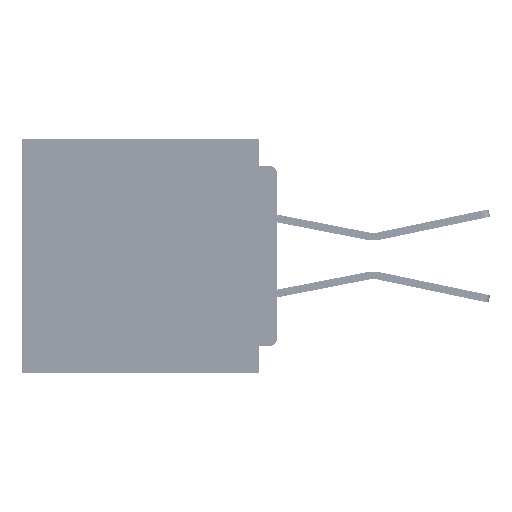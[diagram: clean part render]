
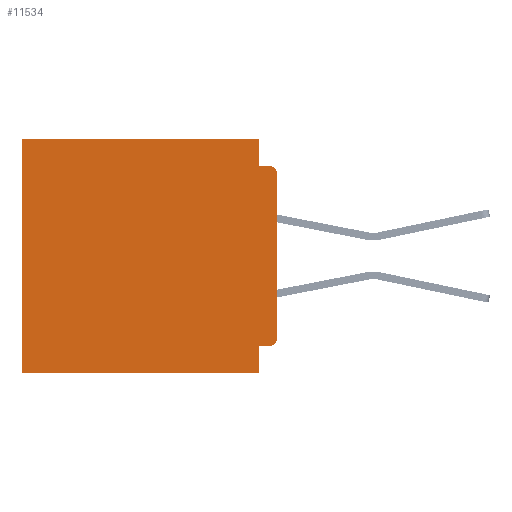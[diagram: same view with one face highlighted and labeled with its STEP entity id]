
A CAD part, left-side view. The second image highlights one B-rep face of the part: STEP entity #11534.
In plain terms, the highlighted planar face has unit normal (-1, 0, 0).
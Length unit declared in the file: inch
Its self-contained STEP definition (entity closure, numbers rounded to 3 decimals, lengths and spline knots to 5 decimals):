
#200 = EDGE_CURVE ( 'NONE', #4685, #11992, #20546, .T. ) ;
#684 = EDGE_LOOP ( 'NONE', ( #48535, #51566, #18633, #61626, #24352, #9855, #30431, #48589, #23209, #20955 ) ) ;
#1313 = VECTOR ( 'NONE', #10297, 39.37008 ) ;
#1827 = DIRECTION ( 'NONE',  ( 0., 0., -1. ) ) ;
#3111 = VECTOR ( 'NONE', #33358, 39.37008 ) ;
#3542 = VECTOR ( 'NONE', #47711, 39.37008 ) ;
#4681 = DIRECTION ( 'NONE',  ( 0., 0., -1. ) ) ;
#4685 = VERTEX_POINT ( 'NONE', #29439 ) ;
#4768 = CIRCLE ( 'NONE', #56144, 0.015 ) ;
#6121 = CARTESIAN_POINT ( 'NONE',  ( 0.3, 0., -0.355 ) ) ;
#6605 = LINE ( 'NONE', #52611, #3542 ) ;
#6770 = CARTESIAN_POINT ( 'NONE',  ( 0.3, 0.031, -0.4 ) ) ;
#7373 = VECTOR ( 'NONE', #21835, 39.37008 ) ;
#7775 = DIRECTION ( 'NONE',  ( -1., 0., 0. ) ) ;
#8286 = PLANE ( 'NONE',  #23350 ) ;
#9855 = ORIENTED_EDGE ( 'NONE', *, *, #56102, .T. ) ;
#10297 = DIRECTION ( 'NONE',  ( 0., 1., 0. ) ) ;
#11070 = DIRECTION ( 'NONE',  ( 0., 1., 0. ) ) ;
#11534 = ADVANCED_FACE ( 'NONE', ( #23353 ), #8286, .F. ) ;
#11992 = VERTEX_POINT ( 'NONE', #26551 ) ;
#13251 = DIRECTION ( 'NONE',  ( 0., 0., -1. ) ) ;
#17113 = VECTOR ( 'NONE', #4681, 39.37008 ) ;
#18633 = ORIENTED_EDGE ( 'NONE', *, *, #31540, .F. ) ;
#18868 = EDGE_CURVE ( 'NONE', #61785, #51885, #62265, .T. ) ;
#19037 = CARTESIAN_POINT ( 'NONE',  ( 0.3, 0.015, -0.355 ) ) ;
#19326 = VERTEX_POINT ( 'NONE', #39690 ) ;
#20546 = LINE ( 'NONE', #61941, #7373 ) ;
#20955 = ORIENTED_EDGE ( 'NONE', *, *, #57345, .T. ) ;
#21835 = DIRECTION ( 'NONE',  ( 0., 1., 0. ) ) ;
#22957 = DIRECTION ( 'NONE',  ( -1., 0., 0. ) ) ;
#23168 = VECTOR ( 'NONE', #1827, 39.37008 ) ;
#23209 = ORIENTED_EDGE ( 'NONE', *, *, #48322, .F. ) ;
#23350 = AXIS2_PLACEMENT_3D ( 'NONE', #32878, #42712, #13251 ) ;
#23353 = FACE_OUTER_BOUND ( 'NONE', #684, .T. ) ;
#24352 = ORIENTED_EDGE ( 'NONE', *, *, #200, .T. ) ;
#25159 = VERTEX_POINT ( 'NONE', #54789 ) ;
#26551 = CARTESIAN_POINT ( 'NONE',  ( 0.3, 0.437, 0. ) ) ;
#27197 = LINE ( 'NONE', #6121, #51786 ) ;
#28138 = VERTEX_POINT ( 'NONE', #58748 ) ;
#29439 = CARTESIAN_POINT ( 'NONE',  ( 0.3, 0.031, 0. ) ) ;
#30431 = ORIENTED_EDGE ( 'NONE', *, *, #61529, .F. ) ;
#31540 = EDGE_CURVE ( 'NONE', #25159, #48718, #52316, .T. ) ;
#32878 = CARTESIAN_POINT ( 'NONE',  ( 0.3, 0., -0.4 ) ) ;
#33358 = DIRECTION ( 'NONE',  ( 0., -1., 0. ) ) ;
#34223 = CARTESIAN_POINT ( 'NONE',  ( 0.3, 0.031, 0. ) ) ;
#37297 = CARTESIAN_POINT ( 'NONE',  ( 0.3, 0.015, -0.06 ) ) ;
#39300 = CARTESIAN_POINT ( 'NONE',  ( 0.3, 0.015, -0.045 ) ) ;
#39690 = CARTESIAN_POINT ( 'NONE',  ( 0.3, 0.437, -0.4 ) ) ;
#40613 = LINE ( 'NONE', #59213, #1313 ) ;
#42242 = DIRECTION ( 'NONE',  ( 0., 0., -1. ) ) ;
#42439 = CARTESIAN_POINT ( 'NONE',  ( 0.3, 0.437, -0.4 ) ) ;
#42663 = VECTOR ( 'NONE', #52264, 39.37008 ) ;
#42712 = DIRECTION ( 'NONE',  ( 1., 0., 0. ) ) ;
#43287 = LINE ( 'NONE', #34223, #17113 ) ;
#45875 = EDGE_CURVE ( 'NONE', #4685, #25159, #43287, .T. ) ;
#46806 = EDGE_CURVE ( 'NONE', #49219, #48718, #4768, .T. ) ;
#47711 = DIRECTION ( 'NONE',  ( 0., 0., -1. ) ) ;
#48322 = EDGE_CURVE ( 'NONE', #60712, #61785, #27197, .T. ) ;
#48535 = ORIENTED_EDGE ( 'NONE', *, *, #55244, .F. ) ;
#48589 = ORIENTED_EDGE ( 'NONE', *, *, #18868, .F. ) ;
#48718 = VERTEX_POINT ( 'NONE', #39300 ) ;
#49219 = VERTEX_POINT ( 'NONE', #57759 ) ;
#50920 = CARTESIAN_POINT ( 'NONE',  ( 0.3, 0.031, -0.4 ) ) ;
#51566 = ORIENTED_EDGE ( 'NONE', *, *, #46806, .T. ) ;
#51721 = CIRCLE ( 'NONE', #53637, 0.015 ) ;
#51786 = VECTOR ( 'NONE', #11070, 39.37008 ) ;
#51885 = VERTEX_POINT ( 'NONE', #50920 ) ;
#52264 = DIRECTION ( 'NONE',  ( 0., 0., -1. ) ) ;
#52316 = LINE ( 'NONE', #57700, #3111 ) ;
#52351 = CARTESIAN_POINT ( 'NONE',  ( 0.3, 0.015, -0.34 ) ) ;
#52611 = CARTESIAN_POINT ( 'NONE',  ( 0.3, 0., -0.4 ) ) ;
#53637 = AXIS2_PLACEMENT_3D ( 'NONE', #52351, #22957, #57220 ) ;
#54789 = CARTESIAN_POINT ( 'NONE',  ( 0.3, 0.031, -0.045 ) ) ;
#55244 = EDGE_CURVE ( 'NONE', #49219, #28138, #6605, .T. ) ;
#55645 = LINE ( 'NONE', #42439, #42663 ) ;
#56102 = EDGE_CURVE ( 'NONE', #11992, #19326, #55645, .T. ) ;
#56144 = AXIS2_PLACEMENT_3D ( 'NONE', #37297, #7775, #42242 ) ;
#57220 = DIRECTION ( 'NONE',  ( 0., 0., -1. ) ) ;
#57345 = EDGE_CURVE ( 'NONE', #60712, #28138, #51721, .T. ) ;
#57700 = CARTESIAN_POINT ( 'NONE',  ( 0.3, 0., -0.045 ) ) ;
#57759 = CARTESIAN_POINT ( 'NONE',  ( 0.3, 0., -0.06 ) ) ;
#58748 = CARTESIAN_POINT ( 'NONE',  ( 0.3, 0., -0.34 ) ) ;
#59213 = CARTESIAN_POINT ( 'NONE',  ( 0.3, 0., -0.4 ) ) ;
#60712 = VERTEX_POINT ( 'NONE', #19037 ) ;
#61384 = CARTESIAN_POINT ( 'NONE',  ( 0.3, 0.031, -0.355 ) ) ;
#61529 = EDGE_CURVE ( 'NONE', #51885, #19326, #40613, .T. ) ;
#61626 = ORIENTED_EDGE ( 'NONE', *, *, #45875, .F. ) ;
#61785 = VERTEX_POINT ( 'NONE', #61384 ) ;
#61941 = CARTESIAN_POINT ( 'NONE',  ( 0.3, 0., 0. ) ) ;
#62265 = LINE ( 'NONE', #6770, #23168 ) ;
